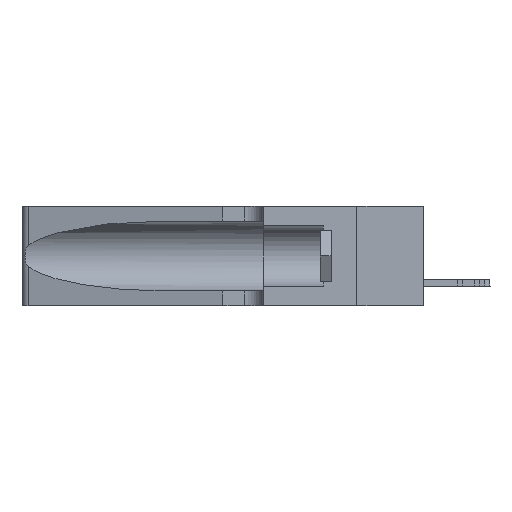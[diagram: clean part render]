
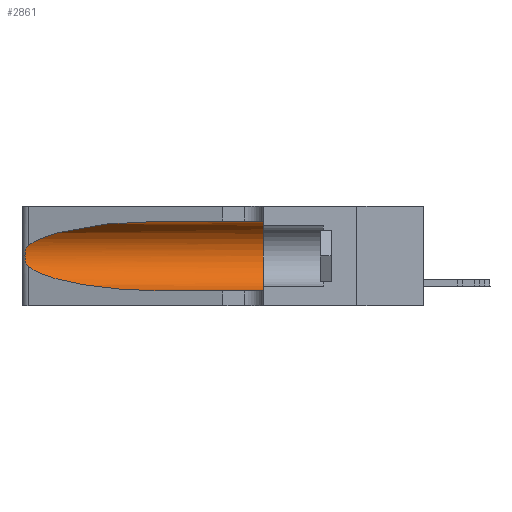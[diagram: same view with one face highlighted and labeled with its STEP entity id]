
A CAD part, left-side view. The second image highlights one B-rep face of the part: STEP entity #2861.
In plain terms, the highlighted cylindrical face has radius 3.308 mm (diameter 6.617 mm), a partial arc.
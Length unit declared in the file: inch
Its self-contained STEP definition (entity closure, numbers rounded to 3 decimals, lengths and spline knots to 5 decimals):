
#1634 = CARTESIAN_POINT ( 'NONE',  ( 0.25639, 1.23184, 0.21858 ) ) ;
#1663 = CIRCLE ( 'NONE', #26643, 0.13025 ) ;
#2861 = ADVANCED_FACE ( 'NONE', ( #20553 ), #48099, .F. ) ;
#3213 = CARTESIAN_POINT ( 'NONE',  ( 0.1305, 0.72297, 0.31525 ) ) ;
#3370 = VERTEX_POINT ( 'NONE', #39872 ) ;
#4420 =( BOUNDED_CURVE ( )  B_SPLINE_CURVE ( 3, ( #3213, #14466, #40882, #33654 ),
 .UNSPECIFIED., .F., .F. ) 
 B_SPLINE_CURVE_WITH_KNOTS ( ( 4, 4 ),
 ( 1.5708, 2.84003 ),
 .UNSPECIFIED. ) 
 CURVE ( )  GEOMETRIC_REPRESENTATION_ITEM ( )  RATIONAL_B_SPLINE_CURVE ( ( 1., 0.87, 0.87, 1. ) ) 
 REPRESENTATION_ITEM ( '' )  );
#4494 = CARTESIAN_POINT ( 'NONE',  ( 0.1305, 0.72297, 0.31525 ) ) ;
#4901 = CARTESIAN_POINT ( 'NONE',  ( 0.25787, 1.23484, 0.2124 ) ) ;
#5909 =( BOUNDED_CURVE ( )  B_SPLINE_CURVE ( 3, ( #47453, #28655, #28487, #39977 ),
 .UNSPECIFIED., .F., .T. ) 
 B_SPLINE_CURVE_WITH_KNOTS ( ( 4, 4 ),
 ( 3.44316, 4.71239 ),
 .UNSPECIFIED. ) 
 CURVE ( )  GEOMETRIC_REPRESENTATION_ITEM ( )  RATIONAL_B_SPLINE_CURVE ( ( 1., 0.87, 0.87, 1. ) ) 
 REPRESENTATION_ITEM ( '' )  );
#8075 = EDGE_LOOP ( 'NONE', ( #18050, #35678, #13068, #20977, #14759, #41144 ) ) ;
#9084 = DIRECTION ( 'NONE',  ( 0., -1., 0. ) ) ;
#10241 = VERTEX_POINT ( 'NONE', #43467 ) ;
#10381 = B_SPLINE_CURVE_WITH_KNOTS ( 'NONE', 3,
 ( #45975, #27353, #1634, #4901, #34560, #34896, #12733, #16345, #30946, #39001, #27830, #42563, #23715, #34731 ),
 .UNSPECIFIED., .F., .F.,
 ( 4, 2, 2, 2, 2, 2, 4 ),
 ( 0., 0.00027, 0.00053, 0.00107, 0.0016, 0.00187, 0.00214 ),
 .UNSPECIFIED. ) ;
#10393 = VERTEX_POINT ( 'NONE', #12244 ) ;
#11589 = VECTOR ( 'NONE', #48407, 39.37008 ) ;
#12007 = DIRECTION ( 'NONE',  ( 0., 0., -1. ) ) ;
#12244 = CARTESIAN_POINT ( 'NONE',  ( 0.1305, 0.35, 0.31525 ) ) ;
#12733 = CARTESIAN_POINT ( 'NONE',  ( 0.26075, 1.23896, 0.19203 ) ) ;
#13068 = ORIENTED_EDGE ( 'NONE', *, *, #46483, .T. ) ;
#14466 = CARTESIAN_POINT ( 'NONE',  ( 0.18966, 0.96281, 0.31525 ) ) ;
#14759 = ORIENTED_EDGE ( 'NONE', *, *, #33636, .F. ) ;
#14980 = DIRECTION ( 'NONE',  ( 0., 0., 1. ) ) ;
#15929 = LINE ( 'NONE', #25995, #26541 ) ;
#16345 = CARTESIAN_POINT ( 'NONE',  ( 0.26075, 1.23896, 0.178 ) ) ;
#18050 = ORIENTED_EDGE ( 'NONE', *, *, #43685, .T. ) ;
#18415 = VERTEX_POINT ( 'NONE', #4494 ) ;
#18850 = CARTESIAN_POINT ( 'NONE',  ( 0.1305, 0.35, 0.05475 ) ) ;
#18939 = CARTESIAN_POINT ( 'NONE',  ( 0.1305, 0.35, 0.185 ) ) ;
#20553 = FACE_OUTER_BOUND ( 'NONE', #8075, .T. ) ;
#20977 = ORIENTED_EDGE ( 'NONE', *, *, #43610, .T. ) ;
#21348 = VERTEX_POINT ( 'NONE', #18850 ) ;
#22214 = CARTESIAN_POINT ( 'NONE',  ( 0.1305, 1.61858, 0.31525 ) ) ;
#23715 = CARTESIAN_POINT ( 'NONE',  ( 0.25555, 1.22993, 0.14849 ) ) ;
#25995 = CARTESIAN_POINT ( 'NONE',  ( 0.1305, 1.61858, 0.05475 ) ) ;
#26541 = VECTOR ( 'NONE', #29744, 39.37008 ) ;
#26643 = AXIS2_PLACEMENT_3D ( 'NONE', #18939, #33368, #14980 ) ;
#27353 = CARTESIAN_POINT ( 'NONE',  ( 0.25555, 1.22994, 0.2215 ) ) ;
#27830 = CARTESIAN_POINT ( 'NONE',  ( 0.25789, 1.23486, 0.15765 ) ) ;
#28487 = CARTESIAN_POINT ( 'NONE',  ( 0.18966, 0.96281, 0.05475 ) ) ;
#28655 = CARTESIAN_POINT ( 'NONE',  ( 0.2373, 1.15595, 0.08982 ) ) ;
#29744 = DIRECTION ( 'NONE',  ( 0., -1., 0. ) ) ;
#30946 = CARTESIAN_POINT ( 'NONE',  ( 0.26017, 1.23833, 0.17102 ) ) ;
#31233 = EDGE_CURVE ( 'NONE', #18415, #10393, #38025, .T. ) ;
#33368 = DIRECTION ( 'NONE',  ( 0., 1., 0. ) ) ;
#33636 = EDGE_CURVE ( 'NONE', #10393, #21348, #1663, .T. ) ;
#33654 = CARTESIAN_POINT ( 'NONE',  ( 0.25487, 1.22718, 0.22369 ) ) ;
#34560 = CARTESIAN_POINT ( 'NONE',  ( 0.25854, 1.2359, 0.20912 ) ) ;
#34731 = CARTESIAN_POINT ( 'NONE',  ( 0.25487, 1.22718, 0.14631 ) ) ;
#34896 = CARTESIAN_POINT ( 'NONE',  ( 0.26018, 1.23835, 0.19895 ) ) ;
#35678 = ORIENTED_EDGE ( 'NONE', *, *, #42525, .T. ) ;
#38025 = LINE ( 'NONE', #22214, #11589 ) ;
#38652 = VERTEX_POINT ( 'NONE', #40645 ) ;
#39001 = CARTESIAN_POINT ( 'NONE',  ( 0.25856, 1.23593, 0.16098 ) ) ;
#39872 = CARTESIAN_POINT ( 'NONE',  ( 0.25487, 1.22718, 0.22369 ) ) ;
#39977 = CARTESIAN_POINT ( 'NONE',  ( 0.1305, 0.72297, 0.05475 ) ) ;
#40645 = CARTESIAN_POINT ( 'NONE',  ( 0.1305, 0.72297, 0.05475 ) ) ;
#40882 = CARTESIAN_POINT ( 'NONE',  ( 0.2373, 1.15595, 0.28018 ) ) ;
#41144 = ORIENTED_EDGE ( 'NONE', *, *, #31233, .F. ) ;
#42525 = EDGE_CURVE ( 'NONE', #3370, #10241, #10381, .T. ) ;
#42563 = CARTESIAN_POINT ( 'NONE',  ( 0.25639, 1.23186, 0.15144 ) ) ;
#43326 = AXIS2_PLACEMENT_3D ( 'NONE', #46406, #9084, #12007 ) ;
#43467 = CARTESIAN_POINT ( 'NONE',  ( 0.25487, 1.22718, 0.14631 ) ) ;
#43610 = EDGE_CURVE ( 'NONE', #38652, #21348, #15929, .T. ) ;
#43685 = EDGE_CURVE ( 'NONE', #18415, #3370, #4420, .T. ) ;
#45975 = CARTESIAN_POINT ( 'NONE',  ( 0.25487, 1.22718, 0.22369 ) ) ;
#46406 = CARTESIAN_POINT ( 'NONE',  ( 0.1305, 1.61858, 0.185 ) ) ;
#46483 = EDGE_CURVE ( 'NONE', #10241, #38652, #5909, .T. ) ;
#47453 = CARTESIAN_POINT ( 'NONE',  ( 0.25487, 1.22718, 0.14631 ) ) ;
#48099 = CYLINDRICAL_SURFACE ( 'NONE', #43326, 0.13025 ) ;
#48407 = DIRECTION ( 'NONE',  ( 0., -1., 0. ) ) ;
